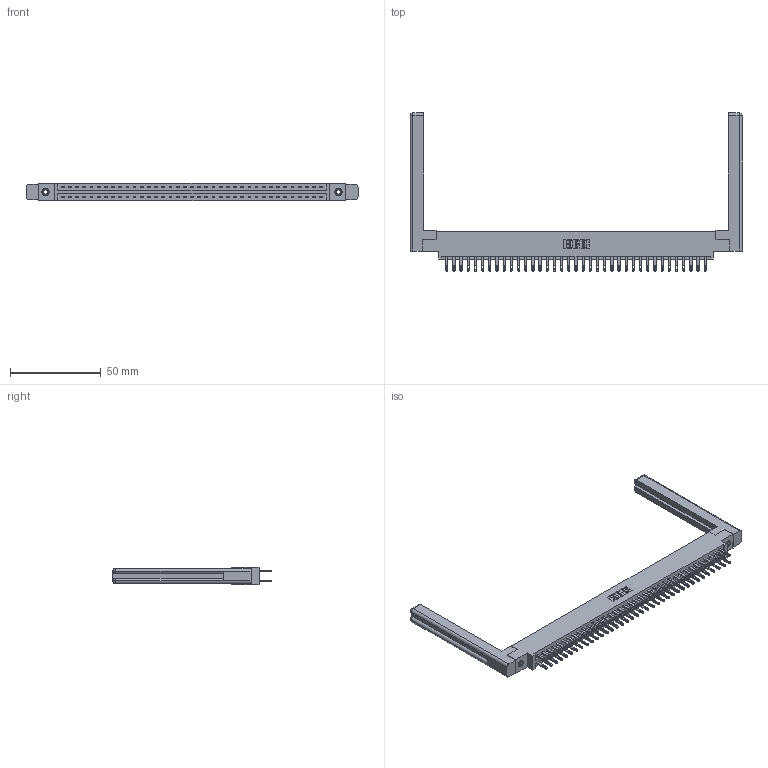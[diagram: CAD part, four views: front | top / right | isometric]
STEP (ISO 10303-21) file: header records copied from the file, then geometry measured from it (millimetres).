
FILE_DESCRIPTION (( 'STEP AP203' ), '1' );
FILE_NAME ('337-074-500-858.STEP', '2019-10-15T12:11:06', ( '' ), ( '' ), 'SwSTEP 2.0', 'SolidWorks 2016', '' );
FILE_SCHEMA (( 'CONFIG_CONTROL_DESIGN' ));
Length unit declared in the file: inch
Products named in the file (5): 345-250-001_345-250-001-102; 337 Part_0.170 Offset - 0.156 Dia-TI; 307-220-058; 345-292-001_345-293-100; 337-074-500-858
Assembly tree (79 placements, depth 2):
  337-074-500-858
    337 Part_0.170 Offset - 0.156 Dia-TI
    345-292-001_345-293-100  x74
    345-250-001_345-250-001-102  x2
    307-220-058  x2
Bounding box: 183.24 x 87.25 x 9.4 mm (x, y, z)
Volume: 26495.2 mm3; surface area: 27805.6 mm2
Topology: 79 solids, 79 shells, 3960 faces, 11999 edges, 7986 vertices
Faces by surface type: plane 2526, cylinder 1410, cone 12, torus 12
Entity records: 32030 total; most frequent: CARTESIAN_POINT 5409, ORIENTED_EDGE 5284, DIRECTION 4626, EDGE_CURVE 2642, VECTOR 2462, LINE 2462, VERTEX_POINT 1754, AXIS2_PLACEMENT_3D 1082
